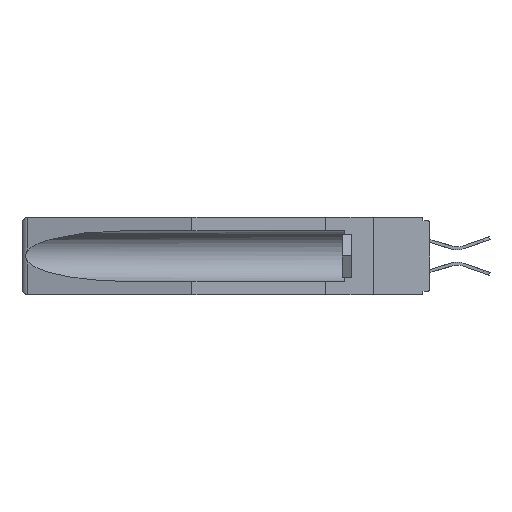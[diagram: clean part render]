
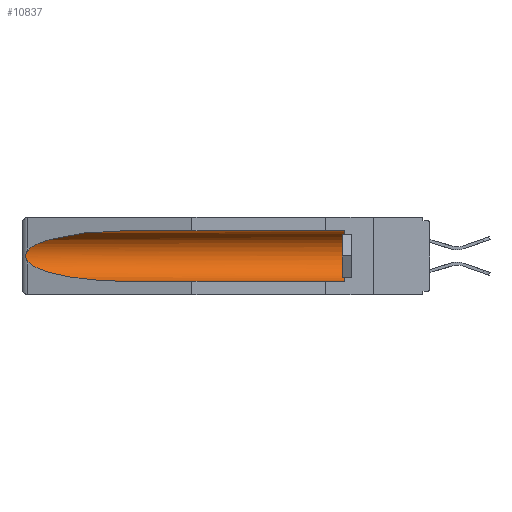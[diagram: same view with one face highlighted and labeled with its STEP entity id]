
A CAD part, left-side view. The second image highlights one B-rep face of the part: STEP entity #10837.
In plain terms, the highlighted cylindrical face has radius 2.857 mm (diameter 5.715 mm), a partial arc.
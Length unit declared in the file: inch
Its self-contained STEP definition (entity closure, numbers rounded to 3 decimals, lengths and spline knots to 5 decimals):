
#135 = CARTESIAN_POINT ( 'NONE',  ( 0.25451, 1.48313, -0.09465 ) ) ;
#336 = CARTESIAN_POINT ( 'NONE',  ( 0.155, -0.30754, -0.284 ) ) ;
#944 = CARTESIAN_POINT ( 'NONE',  ( 0.155, 1.07973, -0.284 ) ) ;
#1409 = CARTESIAN_POINT ( 'NONE',  ( 0.26537, 1.52718, -0.19328 ) ) ;
#1628 =( BOUNDED_CURVE ( )  B_SPLINE_CURVE ( 3, ( #10699, #24480, #12728, #944 ),
 .UNSPECIFIED., .F., .F. ) 
 B_SPLINE_CURVE_WITH_KNOTS ( ( 4, 4 ),
 ( 0.1948, 1.5708 ),
 .UNSPECIFIED. ) 
 CURVE ( )  GEOMETRIC_REPRESENTATION_ITEM ( )  RATIONAL_B_SPLINE_CURVE ( ( 1., 0.848, 0.848, 1. ) ) 
 REPRESENTATION_ITEM ( '' )  );
#1671 = EDGE_CURVE ( 'NONE', #19759, #25102, #14472, .T. ) ;
#2074 = ORIENTED_EDGE ( 'NONE', *, *, #3251, .T. ) ;
#2718 = CARTESIAN_POINT ( 'NONE',  ( 0.26537, 1.52718, -0.14972 ) ) ;
#3235 = CARTESIAN_POINT ( 'NONE',  ( 0.2673, 1.53269, -0.17917 ) ) ;
#3251 = EDGE_CURVE ( 'NONE', #15623, #19759, #21325, .T. ) ;
#3325 = CARTESIAN_POINT ( 'NONE',  ( 0.26654, 1.53092, -0.15636 ) ) ;
#4945 = VERTEX_POINT ( 'NONE', #13311 ) ;
#5068 = CARTESIAN_POINT ( 'NONE',  ( 0.26597, 1.52961, -0.15275 ) ) ;
#5539 = CARTESIAN_POINT ( 'NONE',  ( 0.155, -0.30754, -0.1715 ) ) ;
#6522 = EDGE_CURVE ( 'NONE', #25371, #4945, #1628, .T. ) ;
#6755 = CARTESIAN_POINT ( 'NONE',  ( 0.155, 0.126, -0.059 ) ) ;
#6840 = DIRECTION ( 'NONE',  ( 0., 0., 1. ) ) ;
#7752 = CYLINDRICAL_SURFACE ( 'NONE', #24687, 0.1125 ) ;
#8478 = AXIS2_PLACEMENT_3D ( 'NONE', #14475, #12832, #6840 ) ;
#9075 = VECTOR ( 'NONE', #21929, 39.37008 ) ;
#9138 = VERTEX_POINT ( 'NONE', #18227 ) ;
#10193 = VECTOR ( 'NONE', #13630, 39.37008 ) ;
#10699 = CARTESIAN_POINT ( 'NONE',  ( 0.26537, 1.52718, -0.19328 ) ) ;
#10837 = ADVANCED_FACE ( 'NONE', ( #23395 ), #7752, .F. ) ;
#10920 = CARTESIAN_POINT ( 'NONE',  ( 0.2675, 1.53308, -0.16763 ) ) ;
#10921 = CARTESIAN_POINT ( 'NONE',  ( 0.155, 1.07973, -0.059 ) ) ;
#11079 = CARTESIAN_POINT ( 'NONE',  ( 0.26597, 1.5296, -0.19026 ) ) ;
#12140 = LINE ( 'NONE', #336, #9075 ) ;
#12398 = CARTESIAN_POINT ( 'NONE',  ( 0.155, 1.07973, -0.059 ) ) ;
#12728 = CARTESIAN_POINT ( 'NONE',  ( 0.21114, 1.30732, -0.284 ) ) ;
#12832 = DIRECTION ( 'NONE',  ( 0., -1., 0. ) ) ;
#13192 = CARTESIAN_POINT ( 'NONE',  ( 0.2673, 1.5327, -0.16383 ) ) ;
#13311 = CARTESIAN_POINT ( 'NONE',  ( 0.155, 1.07973, -0.284 ) ) ;
#13630 = DIRECTION ( 'NONE',  ( 0., 1., 0. ) ) ;
#14472 = LINE ( 'NONE', #21882, #10193 ) ;
#14475 = CARTESIAN_POINT ( 'NONE',  ( 0.155, 0.126, -0.1715 ) ) ;
#15197 = CARTESIAN_POINT ( 'NONE',  ( 0.26537, 1.52718, -0.19328 ) ) ;
#15623 = VERTEX_POINT ( 'NONE', #20786 ) ;
#17242 = EDGE_CURVE ( 'NONE', #15623, #4945, #12140, .T. ) ;
#17734 = CARTESIAN_POINT ( 'NONE',  ( 0.21114, 1.30732, -0.059 ) ) ;
#18227 = CARTESIAN_POINT ( 'NONE',  ( 0.26537, 1.52718, -0.14972 ) ) ;
#18879 = CARTESIAN_POINT ( 'NONE',  ( 0.2675, 1.53308, -0.17534 ) ) ;
#18963 = CARTESIAN_POINT ( 'NONE',  ( 0.26655, 1.53094, -0.18657 ) ) ;
#19759 = VERTEX_POINT ( 'NONE', #6755 ) ;
#20028 = CARTESIAN_POINT ( 'NONE',  ( 0.26537, 1.52718, -0.14972 ) ) ;
#20600 = EDGE_CURVE ( 'NONE', #25102, #9138, #25270, .T. ) ;
#20719 = B_SPLINE_CURVE_WITH_KNOTS ( 'NONE', 3,
 ( #2718, #5068, #3325, #13192, #10920, #18879, #3235, #18963, #11079, #1409 ),
 .UNSPECIFIED., .F., .F.,
 ( 4, 2, 2, 2, 4 ),
 ( 0., 0.00029, 0.00058, 0.00087, 0.00117 ),
 .UNSPECIFIED. ) ;
#20786 = CARTESIAN_POINT ( 'NONE',  ( 0.155, 0.126, -0.284 ) ) ;
#20873 = EDGE_LOOP ( 'NONE', ( #24906, #21956, #25003, #25024, #2074, #22115 ) ) ;
#21325 = CIRCLE ( 'NONE', #8478, 0.1125 ) ;
#21882 = CARTESIAN_POINT ( 'NONE',  ( 0.155, -0.30754, -0.059 ) ) ;
#21929 = DIRECTION ( 'NONE',  ( 0., 1., 0. ) ) ;
#21956 = ORIENTED_EDGE ( 'NONE', *, *, #22936, .T. ) ;
#22115 = ORIENTED_EDGE ( 'NONE', *, *, #1671, .T. ) ;
#22936 = EDGE_CURVE ( 'NONE', #9138, #25371, #20719, .T. ) ;
#23202 = DIRECTION ( 'NONE',  ( 0., 1., 0. ) ) ;
#23395 = FACE_OUTER_BOUND ( 'NONE', #20873, .T. ) ;
#24480 = CARTESIAN_POINT ( 'NONE',  ( 0.25451, 1.48313, -0.24835 ) ) ;
#24687 = AXIS2_PLACEMENT_3D ( 'NONE', #5539, #23202, #25292 ) ;
#24906 = ORIENTED_EDGE ( 'NONE', *, *, #20600, .T. ) ;
#25003 = ORIENTED_EDGE ( 'NONE', *, *, #6522, .T. ) ;
#25024 = ORIENTED_EDGE ( 'NONE', *, *, #17242, .F. ) ;
#25102 = VERTEX_POINT ( 'NONE', #12398 ) ;
#25270 =( BOUNDED_CURVE ( )  B_SPLINE_CURVE ( 3, ( #10921, #17734, #135, #20028 ),
 .UNSPECIFIED., .F., .F. ) 
 B_SPLINE_CURVE_WITH_KNOTS ( ( 4, 4 ),
 ( 4.71239, 6.08839 ),
 .UNSPECIFIED. ) 
 CURVE ( )  GEOMETRIC_REPRESENTATION_ITEM ( )  RATIONAL_B_SPLINE_CURVE ( ( 1., 0.848, 0.848, 1. ) ) 
 REPRESENTATION_ITEM ( '' )  );
#25292 = DIRECTION ( 'NONE',  ( 0., 0., 1. ) ) ;
#25371 = VERTEX_POINT ( 'NONE', #15197 ) ;
